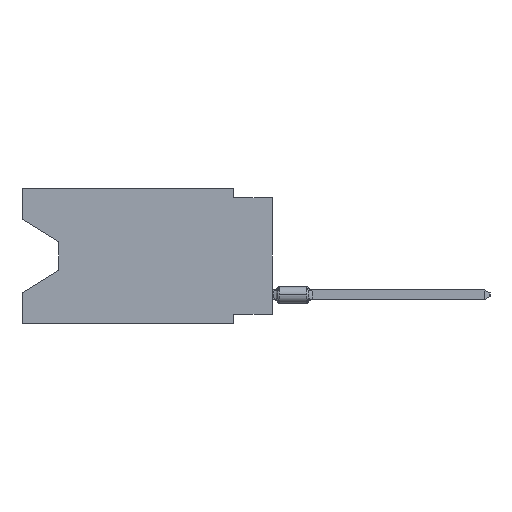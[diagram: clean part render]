
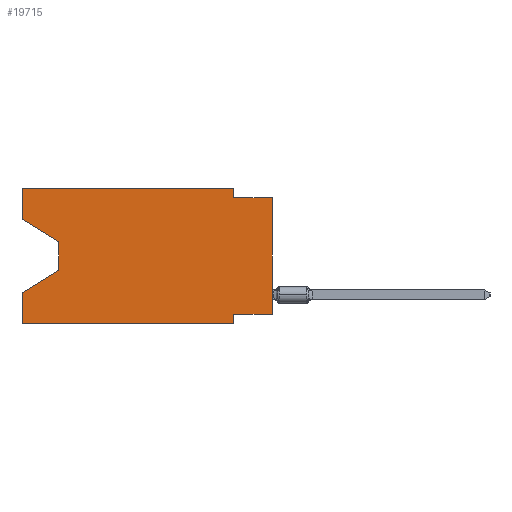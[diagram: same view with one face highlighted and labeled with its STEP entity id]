
A CAD part, left-side view. The second image highlights one B-rep face of the part: STEP entity #19715.
In plain terms, the highlighted planar face has unit normal (-1, 0, 0).
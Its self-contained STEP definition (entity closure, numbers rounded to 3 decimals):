
#67 = LINE ( 'NONE', #8578, #30536 ) ;
#387 = DIRECTION ( 'NONE',  ( 0., -1., 0. ) ) ;
#506 = VECTOR ( 'NONE', #387, 1000. ) ;
#958 = CARTESIAN_POINT ( 'NONE',  ( 0., 16.383, -2.038 ) ) ;
#1014 = CARTESIAN_POINT ( 'NONE',  ( 0., 2.54, -0.635 ) ) ;
#1068 = VECTOR ( 'NONE', #12636, 1000. ) ;
#1834 = CARTESIAN_POINT ( 'NONE',  ( 0., 16.383, 0. ) ) ;
#1885 = VERTEX_POINT ( 'NONE', #18746 ) ;
#1996 = VECTOR ( 'NONE', #29892, 1000. ) ;
#2341 = DIRECTION ( 'NONE',  ( 0., 0., 1. ) ) ;
#2648 = CARTESIAN_POINT ( 'NONE',  ( 0., 16.383, 0. ) ) ;
#2746 = ORIENTED_EDGE ( 'NONE', *, *, #27283, .T. ) ;
#3477 = VERTEX_POINT ( 'NONE', #8812 ) ;
#3937 = CARTESIAN_POINT ( 'NONE',  ( 0., 16.383, 0. ) ) ;
#4039 = ORIENTED_EDGE ( 'NONE', *, *, #8345, .F. ) ;
#4137 = CARTESIAN_POINT ( 'NONE',  ( 0., 16.383, -2.038 ) ) ;
#5001 = CARTESIAN_POINT ( 'NONE',  ( 0., 16.383, 0. ) ) ;
#5885 = CARTESIAN_POINT ( 'NONE',  ( 0., 0., -0.635 ) ) ;
#5920 = CARTESIAN_POINT ( 'NONE',  ( 0., 16.383, 0. ) ) ;
#6009 = LINE ( 'NONE', #30539, #32494 ) ;
#6048 = LINE ( 'NONE', #5885, #506 ) ;
#6072 = EDGE_CURVE ( 'NONE', #11395, #26622, #34912, .T. ) ;
#6931 = LINE ( 'NONE', #30774, #21761 ) ;
#8240 = CARTESIAN_POINT ( 'NONE',  ( 0., 13.97, -5.385 ) ) ;
#8345 = EDGE_CURVE ( 'NONE', #13756, #16594, #29348, .T. ) ;
#8578 = CARTESIAN_POINT ( 'NONE',  ( 0., 13.97, -3.505 ) ) ;
#8812 = CARTESIAN_POINT ( 'NONE',  ( 0., 2.54, -8.255 ) ) ;
#8841 = VECTOR ( 'NONE', #19081, 1000. ) ;
#8961 = EDGE_CURVE ( 'NONE', #25450, #30920, #6009, .T. ) ;
#9146 = CARTESIAN_POINT ( 'NONE',  ( 0., 13.97, -3.505 ) ) ;
#9219 = AXIS2_PLACEMENT_3D ( 'NONE', #2648, #16142, #19347 ) ;
#9735 = EDGE_CURVE ( 'NONE', #3477, #1885, #6931, .T. ) ;
#11233 = ORIENTED_EDGE ( 'NONE', *, *, #32881, .T. ) ;
#11341 = CARTESIAN_POINT ( 'NONE',  ( 0., 0., -8.255 ) ) ;
#11395 = VERTEX_POINT ( 'NONE', #15224 ) ;
#11951 = ORIENTED_EDGE ( 'NONE', *, *, #28522, .F. ) ;
#12636 = DIRECTION ( 'NONE',  ( 0., -0.855, -0.519 ) ) ;
#12934 = CARTESIAN_POINT ( 'NONE',  ( 0., 16.383, -6.852 ) ) ;
#12970 = VECTOR ( 'NONE', #17281, 1000. ) ;
#13756 = VERTEX_POINT ( 'NONE', #958 ) ;
#13899 = DIRECTION ( 'NONE',  ( 0., 0., -1. ) ) ;
#13936 = CARTESIAN_POINT ( 'NONE',  ( 0., 0., 0. ) ) ;
#14012 = EDGE_LOOP ( 'NONE', ( #2746, #14539, #35095, #19584, #11233, #34442, #11951, #34065, #23569, #29792, #32019, #4039 ) ) ;
#14221 = CARTESIAN_POINT ( 'NONE',  ( 0., 16.383, -8.89 ) ) ;
#14348 = DIRECTION ( 'NONE',  ( 0., 0., -1. ) ) ;
#14366 = VECTOR ( 'NONE', #2341, 1000. ) ;
#14539 = ORIENTED_EDGE ( 'NONE', *, *, #31680, .T. ) ;
#15167 = CARTESIAN_POINT ( 'NONE',  ( 0., 0., -0.635 ) ) ;
#15224 = CARTESIAN_POINT ( 'NONE',  ( 0., 13.97, -5.385 ) ) ;
#15399 = EDGE_CURVE ( 'NONE', #33711, #25751, #24086, .T. ) ;
#16142 = DIRECTION ( 'NONE',  ( 1., 0., 0. ) ) ;
#16582 = CARTESIAN_POINT ( 'NONE',  ( 0., 16.383, -8.89 ) ) ;
#16594 = VERTEX_POINT ( 'NONE', #3937 ) ;
#16745 = LINE ( 'NONE', #16582, #28814 ) ;
#17281 = DIRECTION ( 'NONE',  ( 0., -1., 0. ) ) ;
#18746 = CARTESIAN_POINT ( 'NONE',  ( 0., 2.54, -8.89 ) ) ;
#19081 = DIRECTION ( 'NONE',  ( 0., 0.855, -0.519 ) ) ;
#19347 = DIRECTION ( 'NONE',  ( 0., 0., -1. ) ) ;
#19584 = ORIENTED_EDGE ( 'NONE', *, *, #34712, .F. ) ;
#19715 = ADVANCED_FACE ( 'NONE', ( #24513 ), #22013, .F. ) ;
#19860 = VECTOR ( 'NONE', #20680, 1000. ) ;
#20475 = EDGE_CURVE ( 'NONE', #30920, #25751, #6048, .T. ) ;
#20497 = VERTEX_POINT ( 'NONE', #14221 ) ;
#20680 = DIRECTION ( 'NONE',  ( 0., 0., 1. ) ) ;
#21364 = CARTESIAN_POINT ( 'NONE',  ( 0., 0., -8.255 ) ) ;
#21373 = LINE ( 'NONE', #1834, #19860 ) ;
#21761 = VECTOR ( 'NONE', #28633, 1000. ) ;
#22013 = PLANE ( 'NONE',  #9219 ) ;
#22272 = LINE ( 'NONE', #5920, #12970 ) ;
#22296 = DIRECTION ( 'NONE',  ( 0., 0., 1. ) ) ;
#23569 = ORIENTED_EDGE ( 'NONE', *, *, #20475, .F. ) ;
#24086 = LINE ( 'NONE', #13936, #26128 ) ;
#24099 = CARTESIAN_POINT ( 'NONE',  ( 0., 2.54, 0. ) ) ;
#24513 = FACE_OUTER_BOUND ( 'NONE', #14012, .T. ) ;
#24929 = DIRECTION ( 'NONE',  ( 0., -1., 0. ) ) ;
#25450 = VERTEX_POINT ( 'NONE', #24099 ) ;
#25554 = VERTEX_POINT ( 'NONE', #9146 ) ;
#25751 = VERTEX_POINT ( 'NONE', #15167 ) ;
#26128 = VECTOR ( 'NONE', #22296, 1000. ) ;
#26335 = LINE ( 'NONE', #4137, #1068 ) ;
#26622 = VERTEX_POINT ( 'NONE', #12934 ) ;
#27156 = EDGE_CURVE ( 'NONE', #16594, #25450, #22272, .T. ) ;
#27283 = EDGE_CURVE ( 'NONE', #13756, #25554, #26335, .T. ) ;
#28522 = EDGE_CURVE ( 'NONE', #33711, #3477, #29353, .T. ) ;
#28633 = DIRECTION ( 'NONE',  ( 0., 0., -1. ) ) ;
#28814 = VECTOR ( 'NONE', #24929, 1000. ) ;
#29348 = LINE ( 'NONE', #5001, #14366 ) ;
#29353 = LINE ( 'NONE', #21364, #1996 ) ;
#29792 = ORIENTED_EDGE ( 'NONE', *, *, #8961, .F. ) ;
#29892 = DIRECTION ( 'NONE',  ( 0., 1., 0. ) ) ;
#30536 = VECTOR ( 'NONE', #13899, 1000. ) ;
#30539 = CARTESIAN_POINT ( 'NONE',  ( 0., 2.54, 0. ) ) ;
#30774 = CARTESIAN_POINT ( 'NONE',  ( 0., 2.54, -8.89 ) ) ;
#30920 = VERTEX_POINT ( 'NONE', #1014 ) ;
#31680 = EDGE_CURVE ( 'NONE', #25554, #11395, #67, .T. ) ;
#32019 = ORIENTED_EDGE ( 'NONE', *, *, #27156, .F. ) ;
#32494 = VECTOR ( 'NONE', #14348, 1000. ) ;
#32881 = EDGE_CURVE ( 'NONE', #20497, #1885, #16745, .T. ) ;
#33711 = VERTEX_POINT ( 'NONE', #11341 ) ;
#34065 = ORIENTED_EDGE ( 'NONE', *, *, #15399, .T. ) ;
#34442 = ORIENTED_EDGE ( 'NONE', *, *, #9735, .F. ) ;
#34712 = EDGE_CURVE ( 'NONE', #20497, #26622, #21373, .T. ) ;
#34912 = LINE ( 'NONE', #8240, #8841 ) ;
#35095 = ORIENTED_EDGE ( 'NONE', *, *, #6072, .T. ) ;
